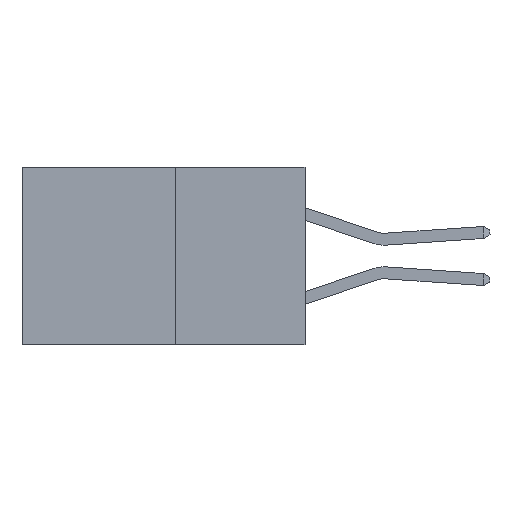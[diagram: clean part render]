
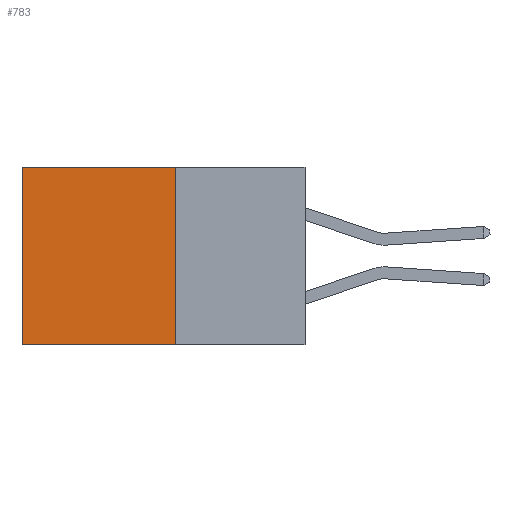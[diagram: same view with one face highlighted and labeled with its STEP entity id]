
A CAD part, left-side view. The second image highlights one B-rep face of the part: STEP entity #783.
In plain terms, the highlighted planar face has unit normal (-1, 0, 0).
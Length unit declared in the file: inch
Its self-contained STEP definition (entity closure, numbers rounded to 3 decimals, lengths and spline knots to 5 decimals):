
#218 = EDGE_CURVE ( 'NONE', #3455, #6965, #2321, .T. ) ;
#478 = LINE ( 'NONE', #5904, #2034 ) ;
#783 = ADVANCED_FACE ( 'NONE', ( #7176 ), #4641, .F. ) ;
#1084 = LINE ( 'NONE', #4867, #5147 ) ;
#1202 = CARTESIAN_POINT ( 'NONE',  ( 0.277, 0.59, 0. ) ) ;
#1357 = CARTESIAN_POINT ( 'NONE',  ( 0.277, 0.59, -0.37 ) ) ;
#1401 = VERTEX_POINT ( 'NONE', #1357 ) ;
#1499 = DIRECTION ( 'NONE',  ( 0., 1., 0. ) ) ;
#2034 = VECTOR ( 'NONE', #4148, 39.37008 ) ;
#2321 = LINE ( 'NONE', #2995, #8129 ) ;
#2834 = CARTESIAN_POINT ( 'NONE',  ( 0.277, 0.27, -0.37 ) ) ;
#2868 = DIRECTION ( 'NONE',  ( 0., 0., -1. ) ) ;
#2995 = CARTESIAN_POINT ( 'NONE',  ( 0.277, 0.27, -0.37 ) ) ;
#3455 = VERTEX_POINT ( 'NONE', #4326 ) ;
#3550 = EDGE_CURVE ( 'NONE', #6965, #1401, #9772, .T. ) ;
#4070 = DIRECTION ( 'NONE',  ( 0., 1., 0. ) ) ;
#4148 = DIRECTION ( 'NONE',  ( 0., 0., -1. ) ) ;
#4256 = ORIENTED_EDGE ( 'NONE', *, *, #218, .F. ) ;
#4326 = CARTESIAN_POINT ( 'NONE',  ( 0.277, 0.27, 0. ) ) ;
#4366 = EDGE_CURVE ( 'NONE', #6770, #1401, #478, .T. ) ;
#4641 = PLANE ( 'NONE',  #8135 ) ;
#4867 = CARTESIAN_POINT ( 'NONE',  ( 0.277, 0.27, 0. ) ) ;
#5147 = VECTOR ( 'NONE', #4070, 39.37008 ) ;
#5245 = CARTESIAN_POINT ( 'NONE',  ( 0.277, 0.27, -0.37 ) ) ;
#5420 = CARTESIAN_POINT ( 'NONE',  ( 0.277, 0.27, -0.37 ) ) ;
#5904 = CARTESIAN_POINT ( 'NONE',  ( 0.277, 0.59, -0.37 ) ) ;
#6028 = VECTOR ( 'NONE', #1499, 39.37008 ) ;
#6494 = ORIENTED_EDGE ( 'NONE', *, *, #4366, .T. ) ;
#6770 = VERTEX_POINT ( 'NONE', #1202 ) ;
#6965 = VERTEX_POINT ( 'NONE', #5420 ) ;
#7176 = FACE_OUTER_BOUND ( 'NONE', #9250, .T. ) ;
#7636 = DIRECTION ( 'NONE',  ( 1., 0., 0. ) ) ;
#8129 = VECTOR ( 'NONE', #9432, 39.37008 ) ;
#8135 = AXIS2_PLACEMENT_3D ( 'NONE', #5245, #7636, #2868 ) ;
#8305 = ORIENTED_EDGE ( 'NONE', *, *, #3550, .F. ) ;
#8850 = EDGE_CURVE ( 'NONE', #3455, #6770, #1084, .T. ) ;
#9250 = EDGE_LOOP ( 'NONE', ( #6494, #8305, #4256, #9783 ) ) ;
#9432 = DIRECTION ( 'NONE',  ( 0., 0., -1. ) ) ;
#9772 = LINE ( 'NONE', #2834, #6028 ) ;
#9783 = ORIENTED_EDGE ( 'NONE', *, *, #8850, .T. ) ;
